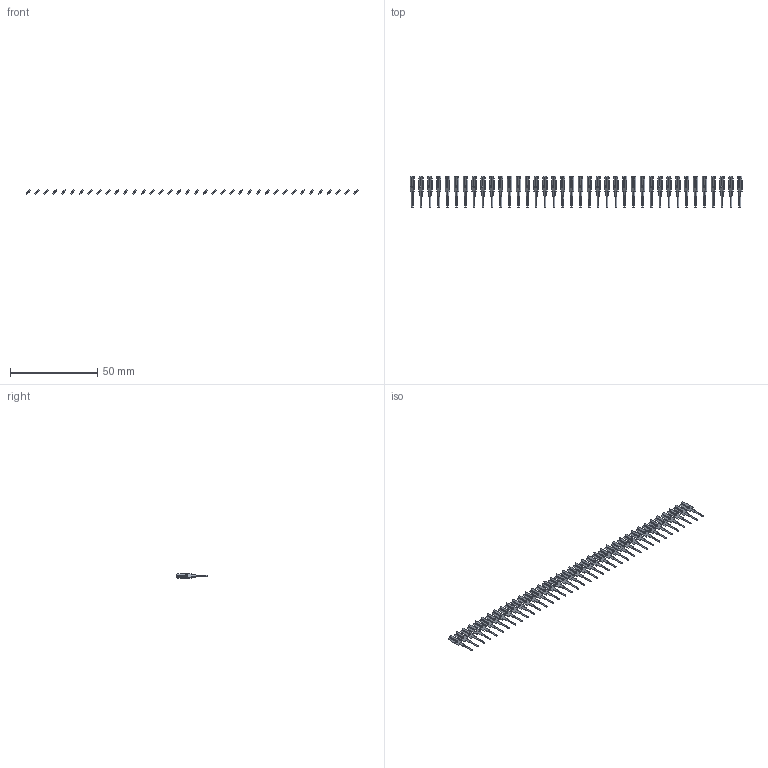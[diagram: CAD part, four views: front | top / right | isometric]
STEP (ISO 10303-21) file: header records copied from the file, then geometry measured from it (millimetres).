
FILE_DESCRIPTION (( 'STEP AP203' ), '1' );
FILE_NAME ('106-038-251-200.STEP', '2020-04-16T19:58:14', ( '' ), ( '' ), 'SwSTEP 2.0', 'SolidWorks 2016', '' );
FILE_SCHEMA (( 'CONFIG_CONTROL_DESIGN' ));
Length unit declared in the file: inch
Products named in the file (2): 100-290-001_100-290-251; 106-038-251-200
Assembly tree (38 placements, depth 2):
  106-038-251-200
    100-290-001_100-290-251  x38
Bounding box: 190.49 x 17.91 x 2.53 mm (x, y, z)
Volume: 694.8 mm3; surface area: 3415 mm2
Topology: 38 solids, 38 shells, 1064 faces, 2964 edges, 1976 vertices
Faces by surface type: plane 836, cylinder 228
Entity records: 2278 total; most frequent: DIRECTION 224, CARTESIAN_POINT 211, ORIENTED_EDGE 156, COORDINATED_UNIVERSAL_TIME_OFFSET 86, LOCAL_TIME 86, CALENDAR_DATE 86, DATE_AND_TIME 86, AXIS2_PLACEMENT_3D 81
